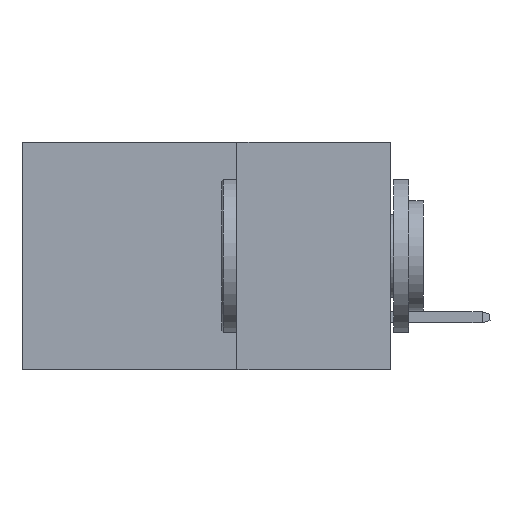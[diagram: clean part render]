
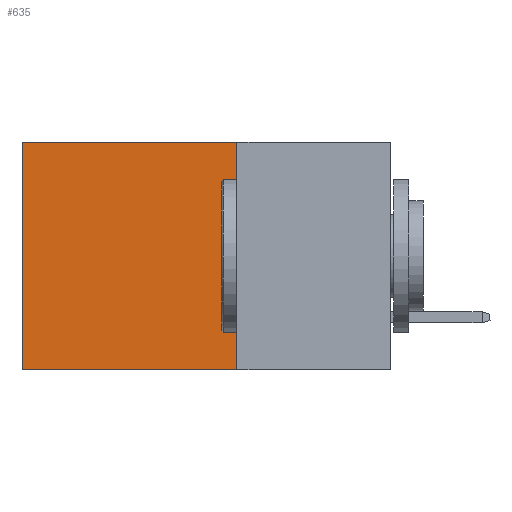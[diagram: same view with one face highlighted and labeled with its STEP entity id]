
A CAD part, left-side view. The second image highlights one B-rep face of the part: STEP entity #635.
In plain terms, the highlighted planar face has unit normal (-1, 0, 0).
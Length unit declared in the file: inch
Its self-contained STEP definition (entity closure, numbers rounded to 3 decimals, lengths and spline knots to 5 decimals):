
#228 = FACE_OUTER_BOUND ( 'NONE', #7564, .T. ) ;
#524 = DIRECTION ( 'NONE',  ( 0., 0., -1. ) ) ;
#601 = DIRECTION ( 'NONE',  ( 1., 0., 0. ) ) ;
#635 = ADVANCED_FACE ( 'NONE', ( #228 ), #8950, .F. ) ;
#835 = LINE ( 'NONE', #4616, #9775 ) ;
#974 = VECTOR ( 'NONE', #1157, 39.37008 ) ;
#1089 = ORIENTED_EDGE ( 'NONE', *, *, #11237, .T. ) ;
#1157 = DIRECTION ( 'NONE',  ( 0., 0., -1. ) ) ;
#1205 = CARTESIAN_POINT ( 'NONE',  ( 0.2875, 0.6, 0. ) ) ;
#1543 = DIRECTION ( 'NONE',  ( 0., 1., 0. ) ) ;
#1589 = EDGE_CURVE ( 'NONE', #2888, #3582, #835, .T. ) ;
#1835 = LINE ( 'NONE', #10956, #8399 ) ;
#2888 = VERTEX_POINT ( 'NONE', #3771 ) ;
#3495 = LINE ( 'NONE', #7580, #7961 ) ;
#3582 = VERTEX_POINT ( 'NONE', #6054 ) ;
#3605 = ORIENTED_EDGE ( 'NONE', *, *, #1589, .F. ) ;
#3771 = CARTESIAN_POINT ( 'NONE',  ( 0.2875, 0.25, -0.37 ) ) ;
#4616 = CARTESIAN_POINT ( 'NONE',  ( 0.2875, 0.25, -0.37 ) ) ;
#4829 = CARTESIAN_POINT ( 'NONE',  ( 0.2875, 0.25, 0. ) ) ;
#5416 = VERTEX_POINT ( 'NONE', #10213 ) ;
#6054 = CARTESIAN_POINT ( 'NONE',  ( 0.2875, 0.6, -0.37 ) ) ;
#6584 = AXIS2_PLACEMENT_3D ( 'NONE', #8151, #601, #8983 ) ;
#6591 = ORIENTED_EDGE ( 'NONE', *, *, #8915, .T. ) ;
#7564 = EDGE_LOOP ( 'NONE', ( #1089, #3605, #8549, #6591 ) ) ;
#7580 = CARTESIAN_POINT ( 'NONE',  ( 0.2875, 0.25, 0. ) ) ;
#7961 = VECTOR ( 'NONE', #8382, 39.37008 ) ;
#8151 = CARTESIAN_POINT ( 'NONE',  ( 0.2875, 0.25, 0. ) ) ;
#8220 = LINE ( 'NONE', #4829, #974 ) ;
#8382 = DIRECTION ( 'NONE',  ( 0., 1., 0. ) ) ;
#8399 = VECTOR ( 'NONE', #524, 39.37008 ) ;
#8549 = ORIENTED_EDGE ( 'NONE', *, *, #8899, .F. ) ;
#8899 = EDGE_CURVE ( 'NONE', #5416, #2888, #8220, .T. ) ;
#8915 = EDGE_CURVE ( 'NONE', #5416, #8940, #3495, .T. ) ;
#8940 = VERTEX_POINT ( 'NONE', #1205 ) ;
#8950 = PLANE ( 'NONE',  #6584 ) ;
#8983 = DIRECTION ( 'NONE',  ( 0., 0., -1. ) ) ;
#9775 = VECTOR ( 'NONE', #1543, 39.37008 ) ;
#10213 = CARTESIAN_POINT ( 'NONE',  ( 0.2875, 0.25, 0. ) ) ;
#10956 = CARTESIAN_POINT ( 'NONE',  ( 0.2875, 0.6, 0. ) ) ;
#11237 = EDGE_CURVE ( 'NONE', #8940, #3582, #1835, .T. ) ;
